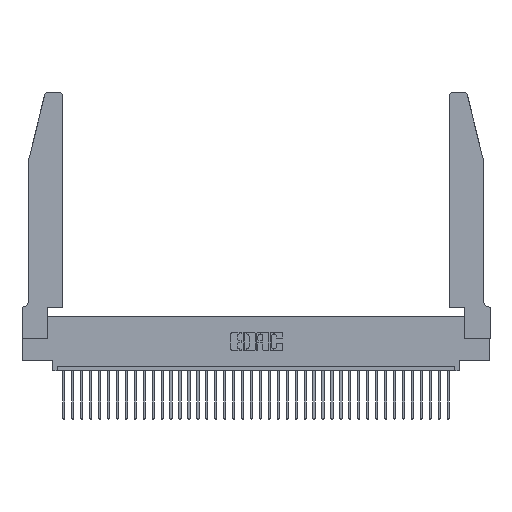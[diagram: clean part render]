
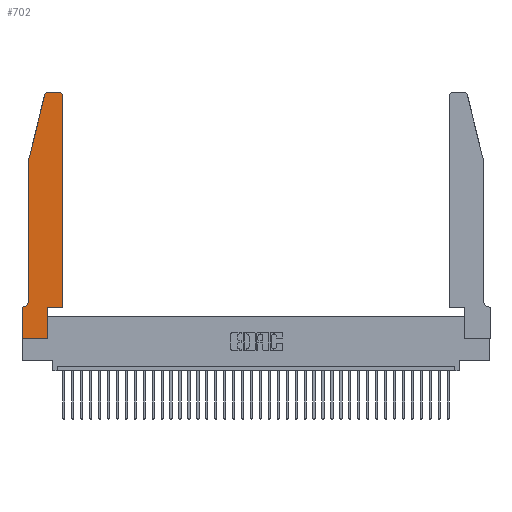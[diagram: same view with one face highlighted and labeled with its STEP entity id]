
A CAD part, top view. The second image highlights one B-rep face of the part: STEP entity #702.
In plain terms, the highlighted planar face has unit normal (0, 0, 1).
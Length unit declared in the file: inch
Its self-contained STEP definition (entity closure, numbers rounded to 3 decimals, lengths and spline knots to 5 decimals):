
#41 = EDGE_CURVE ( 'NONE', #35484, #7698, #8979, .T. ) ;
#702 = ADVANCED_FACE ( 'NONE', ( #13470 ), #20070, .T. ) ;
#1151 = DIRECTION ( 'NONE',  ( 0., 1., 0. ) ) ;
#1460 = LINE ( 'NONE', #36021, #34676 ) ;
#1500 = DIRECTION ( 'NONE',  ( -1., 0., 0. ) ) ;
#2256 = CARTESIAN_POINT ( 'NONE',  ( 0.4205, 2.72, 0.37 ) ) ;
#2291 = CARTESIAN_POINT ( 'NONE',  ( 0.0755, 2., 0.37 ) ) ;
#2437 = CARTESIAN_POINT ( 'NONE',  ( 0.25487, 2.72718, 0.37 ) ) ;
#2456 = DIRECTION ( 'NONE',  ( 0., -1., 0. ) ) ;
#3311 = CARTESIAN_POINT ( 'NONE',  ( 0.2865, 0.35, 0.37 ) ) ;
#3523 = CARTESIAN_POINT ( 'NONE',  ( 0.0755, 0.35, 0.37 ) ) ;
#4743 = DIRECTION ( 'NONE',  ( 0., 0., 1. ) ) ;
#4871 = ORIENTED_EDGE ( 'NONE', *, *, #41, .T. ) ;
#5097 = CIRCLE ( 'NONE', #15141, 0.07 ) ;
#5361 = EDGE_CURVE ( 'NONE', #9520, #36951, #35965, .T. ) ;
#6474 = ORIENTED_EDGE ( 'NONE', *, *, #15143, .T. ) ;
#6794 = VECTOR ( 'NONE', #9384, 39.37008 ) ;
#7052 = DIRECTION ( 'NONE',  ( -1., 0., 0. ) ) ;
#7106 = CARTESIAN_POINT ( 'NONE',  ( 0.284, 2.75, 0.37 ) ) ;
#7250 = ORIENTED_EDGE ( 'NONE', *, *, #8857, .T. ) ;
#7698 = VERTEX_POINT ( 'NONE', #19776 ) ;
#8064 = DIRECTION ( 'NONE',  ( 0., 0., 1. ) ) ;
#8315 = CARTESIAN_POINT ( 'NONE',  ( 0.2605, 2.75, 0.37 ) ) ;
#8324 = CARTESIAN_POINT ( 'NONE',  ( 0., 0.35, 0.37 ) ) ;
#8327 = EDGE_CURVE ( 'NONE', #26473, #13995, #33904, .T. ) ;
#8785 = CARTESIAN_POINT ( 'NONE',  ( 0.0755, 2., 0.37 ) ) ;
#8857 = EDGE_CURVE ( 'NONE', #28211, #10416, #33435, .T. ) ;
#8979 = LINE ( 'NONE', #37127, #9898 ) ;
#9060 = DIRECTION ( 'NONE',  ( -1., 0., 0. ) ) ;
#9384 = DIRECTION ( 'NONE',  ( 1., 0., 0. ) ) ;
#9512 = ORIENTED_EDGE ( 'NONE', *, *, #29590, .T. ) ;
#9520 = VERTEX_POINT ( 'NONE', #2291 ) ;
#9898 = VECTOR ( 'NONE', #28320, 39.37008 ) ;
#10178 = ORIENTED_EDGE ( 'NONE', *, *, #13003, .T. ) ;
#10416 = VERTEX_POINT ( 'NONE', #2437 ) ;
#10568 = CARTESIAN_POINT ( 'NONE',  ( 0.284, 2.72, 0.37 ) ) ;
#11371 = LINE ( 'NONE', #12334, #6794 ) ;
#11769 = VECTOR ( 'NONE', #20779, 39.37008 ) ;
#12334 = CARTESIAN_POINT ( 'NONE',  ( 0., 0., 0.37 ) ) ;
#12616 = CARTESIAN_POINT ( 'NONE',  ( 0., 0.35, 0.37 ) ) ;
#13003 = EDGE_CURVE ( 'NONE', #10416, #9520, #17035, .T. ) ;
#13469 = CARTESIAN_POINT ( 'NONE',  ( 0.4505, 2.72, 0.37 ) ) ;
#13470 = FACE_OUTER_BOUND ( 'NONE', #24509, .T. ) ;
#13995 = VERTEX_POINT ( 'NONE', #18461 ) ;
#14087 = ORIENTED_EDGE ( 'NONE', *, *, #15751, .T. ) ;
#14139 = AXIS2_PLACEMENT_3D ( 'NONE', #10568, #16427, #30964 ) ;
#14640 = AXIS2_PLACEMENT_3D ( 'NONE', #8324, #8064, #16738 ) ;
#14904 = LINE ( 'NONE', #3523, #34064 ) ;
#15141 = AXIS2_PLACEMENT_3D ( 'NONE', #36417, #21994, #7052 ) ;
#15143 = EDGE_CURVE ( 'NONE', #7698, #26473, #1460, .T. ) ;
#15526 = VERTEX_POINT ( 'NONE', #24388 ) ;
#15751 = EDGE_CURVE ( 'NONE', #20473, #27025, #11371, .T. ) ;
#16427 = DIRECTION ( 'NONE',  ( 0., 0., 1. ) ) ;
#16738 = DIRECTION ( 'NONE',  ( 1., 0., 0. ) ) ;
#16814 = ORIENTED_EDGE ( 'NONE', *, *, #21395, .T. ) ;
#16962 = CARTESIAN_POINT ( 'NONE',  ( 0.2865, 0.35, 0.37 ) ) ;
#17035 = LINE ( 'NONE', #26307, #27992 ) ;
#17386 = EDGE_CURVE ( 'NONE', #28552, #20473, #22193, .T. ) ;
#18461 = CARTESIAN_POINT ( 'NONE',  ( 0.4205, 2.75, 0.37 ) ) ;
#18737 = CARTESIAN_POINT ( 'NONE',  ( 0.0755, 0.42, 0.37 ) ) ;
#19293 = LINE ( 'NONE', #8315, #26598 ) ;
#19776 = CARTESIAN_POINT ( 'NONE',  ( 0.4505, 0.35, 0.37 ) ) ;
#19863 = CARTESIAN_POINT ( 'NONE',  ( 0., 0., 0.37 ) ) ;
#20012 = CARTESIAN_POINT ( 'NONE',  ( 0., 0., 0.37 ) ) ;
#20070 = PLANE ( 'NONE',  #14640 ) ;
#20473 = VERTEX_POINT ( 'NONE', #20012 ) ;
#20531 = VECTOR ( 'NONE', #22730, 39.37008 ) ;
#20779 = DIRECTION ( 'NONE',  ( 0., -1., 0. ) ) ;
#21395 = EDGE_CURVE ( 'NONE', #36951, #15526, #5097, .T. ) ;
#21472 = ORIENTED_EDGE ( 'NONE', *, *, #5361, .T. ) ;
#21994 = DIRECTION ( 'NONE',  ( 0., 0., -1. ) ) ;
#22193 = LINE ( 'NONE', #19863, #34492 ) ;
#22730 = DIRECTION ( 'NONE',  ( 0., 1., 0. ) ) ;
#22934 = ORIENTED_EDGE ( 'NONE', *, *, #37392, .T. ) ;
#23396 = DIRECTION ( 'NONE',  ( -0.239, -0.971, 0. ) ) ;
#24388 = CARTESIAN_POINT ( 'NONE',  ( 0.0055, 0.35, 0.37 ) ) ;
#24509 = EDGE_LOOP ( 'NONE', ( #22934, #7250, #10178, #21472, #16814, #35146, #30277, #14087, #9512, #4871, #6474, #26184 ) ) ;
#25543 = LINE ( 'NONE', #16962, #20531 ) ;
#26184 = ORIENTED_EDGE ( 'NONE', *, *, #8327, .T. ) ;
#26307 = CARTESIAN_POINT ( 'NONE',  ( 0.0755, 2., 0.37 ) ) ;
#26473 = VERTEX_POINT ( 'NONE', #13469 ) ;
#26598 = VECTOR ( 'NONE', #9060, 39.37008 ) ;
#27025 = VERTEX_POINT ( 'NONE', #34097 ) ;
#27992 = VECTOR ( 'NONE', #23396, 39.37008 ) ;
#28211 = VERTEX_POINT ( 'NONE', #7106 ) ;
#28320 = DIRECTION ( 'NONE',  ( 1., 0., 0. ) ) ;
#28552 = VERTEX_POINT ( 'NONE', #12616 ) ;
#29590 = EDGE_CURVE ( 'NONE', #27025, #35484, #25543, .T. ) ;
#30276 = AXIS2_PLACEMENT_3D ( 'NONE', #2256, #4743, #34305 ) ;
#30277 = ORIENTED_EDGE ( 'NONE', *, *, #17386, .T. ) ;
#30964 = DIRECTION ( 'NONE',  ( 1., 0., 0. ) ) ;
#33435 = CIRCLE ( 'NONE', #14139, 0.03 ) ;
#33904 = CIRCLE ( 'NONE', #30276, 0.03 ) ;
#34064 = VECTOR ( 'NONE', #1500, 39.37008 ) ;
#34097 = CARTESIAN_POINT ( 'NONE',  ( 0.2865, 0., 0.37 ) ) ;
#34305 = DIRECTION ( 'NONE',  ( 1., 0., 0. ) ) ;
#34492 = VECTOR ( 'NONE', #2456, 39.37008 ) ;
#34676 = VECTOR ( 'NONE', #1151, 39.37008 ) ;
#35146 = ORIENTED_EDGE ( 'NONE', *, *, #36225, .T. ) ;
#35484 = VERTEX_POINT ( 'NONE', #3311 ) ;
#35965 = LINE ( 'NONE', #8785, #11769 ) ;
#36021 = CARTESIAN_POINT ( 'NONE',  ( 0.4505, 0.35, 0.37 ) ) ;
#36225 = EDGE_CURVE ( 'NONE', #15526, #28552, #14904, .T. ) ;
#36417 = CARTESIAN_POINT ( 'NONE',  ( 0.0055, 0.42, 0.37 ) ) ;
#36951 = VERTEX_POINT ( 'NONE', #18737 ) ;
#37127 = CARTESIAN_POINT ( 'NONE',  ( 0.4505, 0.35, 0.37 ) ) ;
#37392 = EDGE_CURVE ( 'NONE', #13995, #28211, #19293, .T. ) ;
